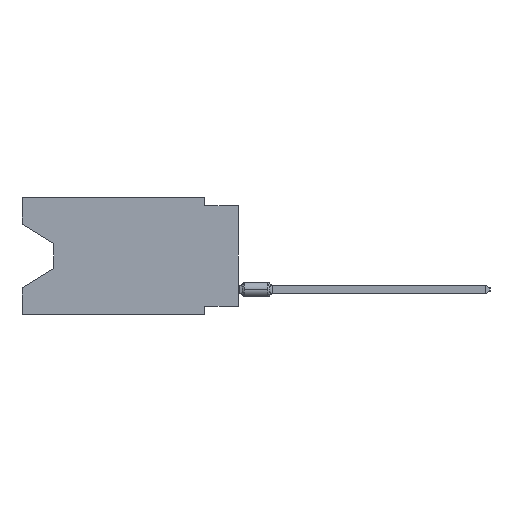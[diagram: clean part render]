
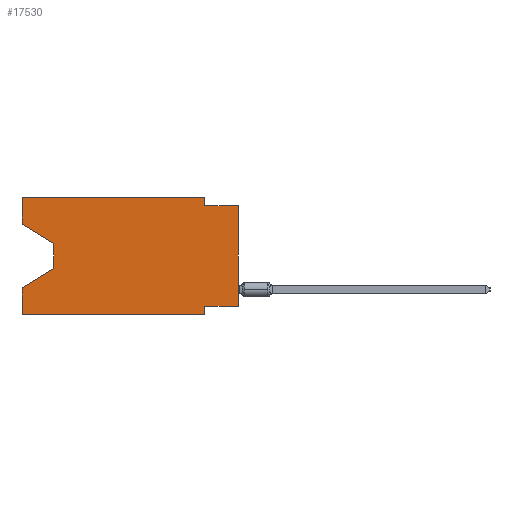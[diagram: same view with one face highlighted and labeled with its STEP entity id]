
A CAD part, left-side view. The second image highlights one B-rep face of the part: STEP entity #17530.
In plain terms, the highlighted planar face has unit normal (-1, 0, 0).
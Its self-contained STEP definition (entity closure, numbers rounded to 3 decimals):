
#522 = CARTESIAN_POINT ( 'NONE',  ( 0., 13.97, -5.385 ) ) ;
#586 = LINE ( 'NONE', #16690, #49015 ) ;
#1412 = CARTESIAN_POINT ( 'NONE',  ( 0., 16.383, -6.852 ) ) ;
#1704 = DIRECTION ( 'NONE',  ( 0., 1., 0. ) ) ;
#2152 = EDGE_CURVE ( 'NONE', #27360, #11535, #43680, .T. ) ;
#2310 = CARTESIAN_POINT ( 'NONE',  ( 0., 2.54, -8.255 ) ) ;
#6818 = LINE ( 'NONE', #28163, #31984 ) ;
#7319 = EDGE_CURVE ( 'NONE', #16801, #10325, #57255, .T. ) ;
#7495 = DIRECTION ( 'NONE',  ( 0., 0., -1. ) ) ;
#9045 = DIRECTION ( 'NONE',  ( 0., 0., -1. ) ) ;
#9080 = EDGE_CURVE ( 'NONE', #16801, #33169, #41022, .T. ) ;
#9366 = DIRECTION ( 'NONE',  ( 0., 0., 1. ) ) ;
#9455 = VERTEX_POINT ( 'NONE', #30394 ) ;
#10074 = CARTESIAN_POINT ( 'NONE',  ( 0., 13.97, -3.505 ) ) ;
#10154 = ORIENTED_EDGE ( 'NONE', *, *, #64395, .F. ) ;
#10325 = VERTEX_POINT ( 'NONE', #1412 ) ;
#10701 = EDGE_CURVE ( 'NONE', #65782, #31856, #63611, .T. ) ;
#11535 = VERTEX_POINT ( 'NONE', #2310 ) ;
#11590 = LINE ( 'NONE', #12614, #69156 ) ;
#12337 = DIRECTION ( 'NONE',  ( 0., 0., 1. ) ) ;
#12614 = CARTESIAN_POINT ( 'NONE',  ( 0., 16.383, -2.038 ) ) ;
#12941 = CARTESIAN_POINT ( 'NONE',  ( 0., 2.54, -8.89 ) ) ;
#14524 = ORIENTED_EDGE ( 'NONE', *, *, #56003, .T. ) ;
#14542 = EDGE_LOOP ( 'NONE', ( #28480, #63587, #51388, #52709, #19795, #48949, #24996, #14524, #10154, #53829, #51990, #31924 ) ) ;
#14563 = LINE ( 'NONE', #522, #52201 ) ;
#14852 = VERTEX_POINT ( 'NONE', #44224 ) ;
#16690 = CARTESIAN_POINT ( 'NONE',  ( 0., 0., 0. ) ) ;
#16801 = VERTEX_POINT ( 'NONE', #47927 ) ;
#16924 = DIRECTION ( 'NONE',  ( 0., -1., 0. ) ) ;
#17081 = DIRECTION ( 'NONE',  ( 0., -1., 0. ) ) ;
#17530 = ADVANCED_FACE ( 'NONE', ( #48485 ), #49841, .F. ) ;
#18656 = CARTESIAN_POINT ( 'NONE',  ( 0., 0., -0.635 ) ) ;
#18838 = CARTESIAN_POINT ( 'NONE',  ( 0., 16.383, 0. ) ) ;
#19795 = ORIENTED_EDGE ( 'NONE', *, *, #9080, .T. ) ;
#19962 = VERTEX_POINT ( 'NONE', #42475 ) ;
#20337 = VERTEX_POINT ( 'NONE', #18656 ) ;
#22498 = CARTESIAN_POINT ( 'NONE',  ( 0., 16.383, 0. ) ) ;
#22783 = DIRECTION ( 'NONE',  ( 0., -0.855, -0.519 ) ) ;
#23045 = CARTESIAN_POINT ( 'NONE',  ( 0., 0., -8.255 ) ) ;
#24996 = ORIENTED_EDGE ( 'NONE', *, *, #2152, .F. ) ;
#27360 = VERTEX_POINT ( 'NONE', #59557 ) ;
#27626 = EDGE_CURVE ( 'NONE', #31856, #9455, #54917, .T. ) ;
#28163 = CARTESIAN_POINT ( 'NONE',  ( 0., 2.54, -8.89 ) ) ;
#28480 = ORIENTED_EDGE ( 'NONE', *, *, #56990, .T. ) ;
#28539 = DIRECTION ( 'NONE',  ( 1., 0., 0. ) ) ;
#29986 = CARTESIAN_POINT ( 'NONE',  ( 0., 2.54, 0. ) ) ;
#30394 = CARTESIAN_POINT ( 'NONE',  ( 0., 2.54, -0.635 ) ) ;
#31856 = VERTEX_POINT ( 'NONE', #29986 ) ;
#31924 = ORIENTED_EDGE ( 'NONE', *, *, #32728, .F. ) ;
#31984 = VECTOR ( 'NONE', #7495, 1000. ) ;
#32197 = VECTOR ( 'NONE', #16924, 1000. ) ;
#32728 = EDGE_CURVE ( 'NONE', #14852, #65782, #50062, .T. ) ;
#33169 = VERTEX_POINT ( 'NONE', #12941 ) ;
#33773 = CARTESIAN_POINT ( 'NONE',  ( 0., 16.383, 0. ) ) ;
#34017 = CARTESIAN_POINT ( 'NONE',  ( 0., 0., -0.635 ) ) ;
#34195 = EDGE_CURVE ( 'NONE', #11535, #33169, #6818, .T. ) ;
#34272 = CARTESIAN_POINT ( 'NONE',  ( 0., 2.54, 0. ) ) ;
#39047 = CARTESIAN_POINT ( 'NONE',  ( 0., 13.97, -5.385 ) ) ;
#39202 = VECTOR ( 'NONE', #9045, 1000. ) ;
#39525 = DIRECTION ( 'NONE',  ( 0., 0., -1. ) ) ;
#40887 = CARTESIAN_POINT ( 'NONE',  ( 0., 16.383, 0. ) ) ;
#41022 = LINE ( 'NONE', #57446, #48667 ) ;
#41369 = DIRECTION ( 'NONE',  ( 0., -1., 0. ) ) ;
#41792 = VECTOR ( 'NONE', #9366, 1000. ) ;
#41954 = CARTESIAN_POINT ( 'NONE',  ( 0., 16.383, 0. ) ) ;
#42475 = CARTESIAN_POINT ( 'NONE',  ( 0., 13.97, -3.505 ) ) ;
#42702 = EDGE_CURVE ( 'NONE', #52868, #10325, #14563, .T. ) ;
#43680 = LINE ( 'NONE', #23045, #55742 ) ;
#44224 = CARTESIAN_POINT ( 'NONE',  ( 0., 16.383, -2.038 ) ) ;
#46516 = EDGE_CURVE ( 'NONE', #19962, #52868, #57969, .T. ) ;
#47927 = CARTESIAN_POINT ( 'NONE',  ( 0., 16.383, -8.89 ) ) ;
#48271 = VECTOR ( 'NONE', #39525, 1000. ) ;
#48433 = DIRECTION ( 'NONE',  ( 0., 0.855, -0.519 ) ) ;
#48485 = FACE_OUTER_BOUND ( 'NONE', #14542, .T. ) ;
#48667 = VECTOR ( 'NONE', #41369, 1000. ) ;
#48949 = ORIENTED_EDGE ( 'NONE', *, *, #34195, .F. ) ;
#49015 = VECTOR ( 'NONE', #59328, 1000. ) ;
#49841 = PLANE ( 'NONE',  #64430 ) ;
#50062 = LINE ( 'NONE', #22498, #53032 ) ;
#51388 = ORIENTED_EDGE ( 'NONE', *, *, #42702, .T. ) ;
#51990 = ORIENTED_EDGE ( 'NONE', *, *, #10701, .F. ) ;
#52201 = VECTOR ( 'NONE', #48433, 1000. ) ;
#52709 = ORIENTED_EDGE ( 'NONE', *, *, #7319, .F. ) ;
#52868 = VERTEX_POINT ( 'NONE', #39047 ) ;
#53032 = VECTOR ( 'NONE', #12337, 1000. ) ;
#53829 = ORIENTED_EDGE ( 'NONE', *, *, #27626, .F. ) ;
#54917 = LINE ( 'NONE', #34272, #48271 ) ;
#55742 = VECTOR ( 'NONE', #1704, 1000. ) ;
#56003 = EDGE_CURVE ( 'NONE', #27360, #20337, #586, .T. ) ;
#56990 = EDGE_CURVE ( 'NONE', #14852, #19962, #11590, .T. ) ;
#57255 = LINE ( 'NONE', #18838, #41792 ) ;
#57446 = CARTESIAN_POINT ( 'NONE',  ( 0., 16.383, -8.89 ) ) ;
#57595 = VECTOR ( 'NONE', #17081, 1000. ) ;
#57969 = LINE ( 'NONE', #10074, #39202 ) ;
#59328 = DIRECTION ( 'NONE',  ( 0., 0., 1. ) ) ;
#59557 = CARTESIAN_POINT ( 'NONE',  ( 0., 0., -8.255 ) ) ;
#59667 = DIRECTION ( 'NONE',  ( 0., 0., -1. ) ) ;
#63587 = ORIENTED_EDGE ( 'NONE', *, *, #46516, .T. ) ;
#63611 = LINE ( 'NONE', #40887, #57595 ) ;
#64395 = EDGE_CURVE ( 'NONE', #9455, #20337, #65512, .T. ) ;
#64430 = AXIS2_PLACEMENT_3D ( 'NONE', #33773, #28539, #59667 ) ;
#65512 = LINE ( 'NONE', #34017, #32197 ) ;
#65782 = VERTEX_POINT ( 'NONE', #41954 ) ;
#69156 = VECTOR ( 'NONE', #22783, 1000. ) ;
